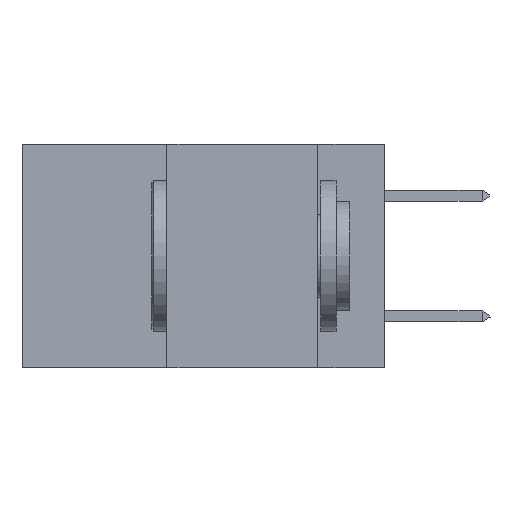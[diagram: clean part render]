
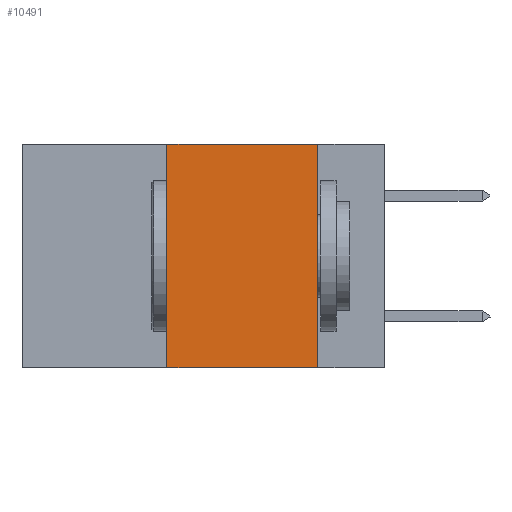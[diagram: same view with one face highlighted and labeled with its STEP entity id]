
A CAD part, left-side view. The second image highlights one B-rep face of the part: STEP entity #10491.
In plain terms, the highlighted planar face has unit normal (-1, 0, 0).
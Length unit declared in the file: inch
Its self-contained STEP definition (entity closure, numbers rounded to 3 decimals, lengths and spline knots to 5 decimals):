
#2255 = LINE ( 'NONE', #16943, #19367 ) ;
#3007 = EDGE_CURVE ( 'NONE', #16896, #9210, #2255, .T. ) ;
#3810 = CARTESIAN_POINT ( 'NONE',  ( 0., 0.6, -0.37 ) ) ;
#3842 = LINE ( 'NONE', #8778, #8764 ) ;
#5415 = CARTESIAN_POINT ( 'NONE',  ( 0., 0.11, -0.37 ) ) ;
#5448 = EDGE_CURVE ( 'NONE', #16386, #12214, #10660, .T. ) ;
#6583 = DIRECTION ( 'NONE',  ( 1., 0., 0. ) ) ;
#6738 = EDGE_LOOP ( 'NONE', ( #16850, #13046, #18536, #12762 ) ) ;
#7120 = FACE_OUTER_BOUND ( 'NONE', #6738, .T. ) ;
#7283 = CARTESIAN_POINT ( 'NONE',  ( 0., 0.11, 0. ) ) ;
#8225 = CARTESIAN_POINT ( 'NONE',  ( 0., 0.6, 0. ) ) ;
#8354 = VECTOR ( 'NONE', #18211, 39.37008 ) ;
#8764 = VECTOR ( 'NONE', #10369, 39.37008 ) ;
#8778 = CARTESIAN_POINT ( 'NONE',  ( 0., 0.36, 0. ) ) ;
#9210 = VERTEX_POINT ( 'NONE', #7283 ) ;
#9325 = LINE ( 'NONE', #13460, #8354 ) ;
#9765 = DIRECTION ( 'NONE',  ( 0., -1., 0. ) ) ;
#10256 = EDGE_CURVE ( 'NONE', #9210, #12214, #9325, .T. ) ;
#10369 = DIRECTION ( 'NONE',  ( 0., 0., 1. ) ) ;
#10487 = CARTESIAN_POINT ( 'NONE',  ( 0., 0.36, 0. ) ) ;
#10491 = ADVANCED_FACE ( 'NONE', ( #7120 ), #12658, .F. ) ;
#10660 = LINE ( 'NONE', #3810, #13088 ) ;
#10827 = DIRECTION ( 'NONE',  ( 0., -1., 0. ) ) ;
#10933 = CARTESIAN_POINT ( 'NONE',  ( 0., 0.36, -0.37 ) ) ;
#12214 = VERTEX_POINT ( 'NONE', #5415 ) ;
#12658 = PLANE ( 'NONE',  #19042 ) ;
#12762 = ORIENTED_EDGE ( 'NONE', *, *, #5448, .T. ) ;
#13046 = ORIENTED_EDGE ( 'NONE', *, *, #3007, .F. ) ;
#13088 = VECTOR ( 'NONE', #9765, 39.37008 ) ;
#13460 = CARTESIAN_POINT ( 'NONE',  ( 0., 0.11, 0. ) ) ;
#14250 = DIRECTION ( 'NONE',  ( 0., 0., -1. ) ) ;
#15227 = EDGE_CURVE ( 'NONE', #16386, #16896, #3842, .T. ) ;
#16386 = VERTEX_POINT ( 'NONE', #10933 ) ;
#16850 = ORIENTED_EDGE ( 'NONE', *, *, #10256, .F. ) ;
#16896 = VERTEX_POINT ( 'NONE', #10487 ) ;
#16943 = CARTESIAN_POINT ( 'NONE',  ( 0., 0.6, 0. ) ) ;
#18211 = DIRECTION ( 'NONE',  ( 0., 0., -1. ) ) ;
#18536 = ORIENTED_EDGE ( 'NONE', *, *, #15227, .F. ) ;
#19042 = AXIS2_PLACEMENT_3D ( 'NONE', #8225, #6583, #14250 ) ;
#19367 = VECTOR ( 'NONE', #10827, 39.37008 ) ;
